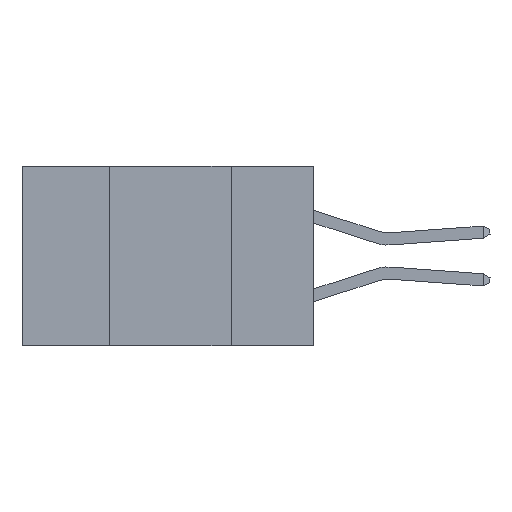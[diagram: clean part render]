
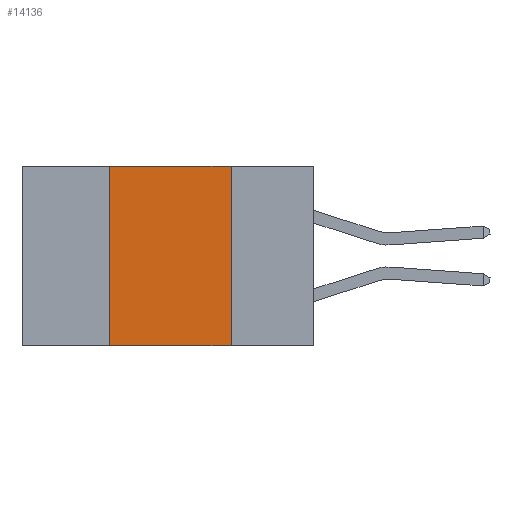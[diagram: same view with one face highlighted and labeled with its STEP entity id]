
A CAD part, left-side view. The second image highlights one B-rep face of the part: STEP entity #14136.
In plain terms, the highlighted planar face has unit normal (-1, 0, 0).
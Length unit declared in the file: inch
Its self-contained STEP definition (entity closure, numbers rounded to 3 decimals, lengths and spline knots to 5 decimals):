
#1380 = PLANE ( 'NONE',  #13335 ) ;
#1742 = DIRECTION ( 'NONE',  ( 0., 0., -1. ) ) ;
#1770 = EDGE_CURVE ( 'NONE', #7775, #18682, #20864, .T. ) ;
#1795 = EDGE_CURVE ( 'NONE', #7775, #12209, #6348, .T. ) ;
#3380 = DIRECTION ( 'NONE',  ( 0., 0., 1. ) ) ;
#4037 = ORIENTED_EDGE ( 'NONE', *, *, #13650, .F. ) ;
#5458 = DIRECTION ( 'NONE',  ( 0., 0., -1. ) ) ;
#5669 = FACE_OUTER_BOUND ( 'NONE', #14327, .T. ) ;
#6348 = LINE ( 'NONE', #22037, #24164 ) ;
#6609 = VECTOR ( 'NONE', #5458, 39.37008 ) ;
#7582 = VECTOR ( 'NONE', #25544, 39.37008 ) ;
#7775 = VERTEX_POINT ( 'NONE', #23635 ) ;
#8275 = LINE ( 'NONE', #18903, #6609 ) ;
#9781 = ORIENTED_EDGE ( 'NONE', *, *, #1795, .F. ) ;
#12209 = VERTEX_POINT ( 'NONE', #34333 ) ;
#13335 = AXIS2_PLACEMENT_3D ( 'NONE', #30437, #33378, #1742 ) ;
#13650 = EDGE_CURVE ( 'NONE', #12209, #16854, #33546, .T. ) ;
#14136 = ADVANCED_FACE ( 'NONE', ( #5669 ), #1380, .F. ) ;
#14327 = EDGE_LOOP ( 'NONE', ( #21806, #4037, #9781, #19998 ) ) ;
#16854 = VERTEX_POINT ( 'NONE', #22861 ) ;
#18682 = VERTEX_POINT ( 'NONE', #33557 ) ;
#18903 = CARTESIAN_POINT ( 'NONE',  ( 0., 0.17, 0. ) ) ;
#19998 = ORIENTED_EDGE ( 'NONE', *, *, #1770, .T. ) ;
#20864 = LINE ( 'NONE', #30682, #7582 ) ;
#21806 = ORIENTED_EDGE ( 'NONE', *, *, #30891, .F. ) ;
#22037 = CARTESIAN_POINT ( 'NONE',  ( 0., 0.42, 0. ) ) ;
#22861 = CARTESIAN_POINT ( 'NONE',  ( 0., 0.17, 0. ) ) ;
#23527 = VECTOR ( 'NONE', #31877, 39.37008 ) ;
#23635 = CARTESIAN_POINT ( 'NONE',  ( 0., 0.42, -0.37 ) ) ;
#23713 = CARTESIAN_POINT ( 'NONE',  ( 0., 0.6, 0. ) ) ;
#24164 = VECTOR ( 'NONE', #3380, 39.37008 ) ;
#25544 = DIRECTION ( 'NONE',  ( 0., -1., 0. ) ) ;
#30437 = CARTESIAN_POINT ( 'NONE',  ( 0., 0.6, 0. ) ) ;
#30682 = CARTESIAN_POINT ( 'NONE',  ( 0., 0.6, -0.37 ) ) ;
#30891 = EDGE_CURVE ( 'NONE', #16854, #18682, #8275, .T. ) ;
#31877 = DIRECTION ( 'NONE',  ( 0., -1., 0. ) ) ;
#33378 = DIRECTION ( 'NONE',  ( 1., 0., 0. ) ) ;
#33546 = LINE ( 'NONE', #23713, #23527 ) ;
#33557 = CARTESIAN_POINT ( 'NONE',  ( 0., 0.17, -0.37 ) ) ;
#34333 = CARTESIAN_POINT ( 'NONE',  ( 0., 0.42, 0. ) ) ;
